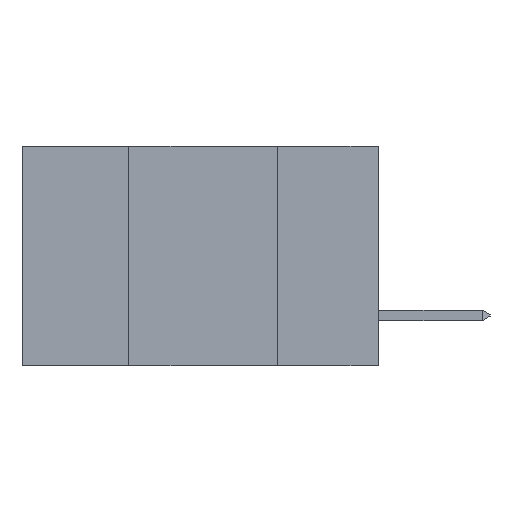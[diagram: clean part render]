
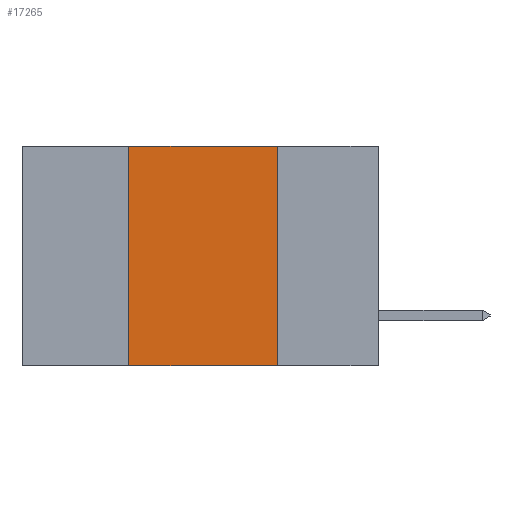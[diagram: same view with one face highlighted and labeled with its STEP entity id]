
A CAD part, left-side view. The second image highlights one B-rep face of the part: STEP entity #17265.
In plain terms, the highlighted planar face has unit normal (-1, 0, 0).
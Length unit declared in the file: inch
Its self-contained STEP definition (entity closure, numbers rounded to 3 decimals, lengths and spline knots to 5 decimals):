
#1045 = ORIENTED_EDGE ( 'NONE', *, *, #14890, .F. ) ;
#1992 = ORIENTED_EDGE ( 'NONE', *, *, #7473, .F. ) ;
#3043 = VECTOR ( 'NONE', #18909, 39.37008 ) ;
#3539 = DIRECTION ( 'NONE',  ( 0., 0., -1. ) ) ;
#3672 = PLANE ( 'NONE',  #11408 ) ;
#6373 = LINE ( 'NONE', #8031, #9972 ) ;
#6906 = CARTESIAN_POINT ( 'NONE',  ( 0., 0.6, 0. ) ) ;
#7210 = ORIENTED_EDGE ( 'NONE', *, *, #8433, .F. ) ;
#7400 = LINE ( 'NONE', #14899, #11900 ) ;
#7473 = EDGE_CURVE ( 'NONE', #14753, #12219, #7400, .T. ) ;
#8031 = CARTESIAN_POINT ( 'NONE',  ( 0., 0.17, -0.37 ) ) ;
#8240 = CARTESIAN_POINT ( 'NONE',  ( 0., 0.6, 0. ) ) ;
#8433 = EDGE_CURVE ( 'NONE', #16001, #8693, #6373, .T. ) ;
#8515 = FACE_OUTER_BOUND ( 'NONE', #13939, .T. ) ;
#8517 = CARTESIAN_POINT ( 'NONE',  ( 0., 0.6, -0.37 ) ) ;
#8693 = VERTEX_POINT ( 'NONE', #8708 ) ;
#8708 = CARTESIAN_POINT ( 'NONE',  ( 0., 0.17, -0.37 ) ) ;
#9569 = VECTOR ( 'NONE', #15900, 39.37008 ) ;
#9775 = DIRECTION ( 'NONE',  ( 0., 0., -1. ) ) ;
#9972 = VECTOR ( 'NONE', #3539, 39.37008 ) ;
#10626 = LINE ( 'NONE', #8517, #3043 ) ;
#11408 = AXIS2_PLACEMENT_3D ( 'NONE', #8240, #18656, #9775 ) ;
#11900 = VECTOR ( 'NONE', #17886, 39.37008 ) ;
#12219 = VERTEX_POINT ( 'NONE', #15940 ) ;
#13939 = EDGE_LOOP ( 'NONE', ( #7210, #1045, #1992, #17986 ) ) ;
#14753 = VERTEX_POINT ( 'NONE', #18864 ) ;
#14890 = EDGE_CURVE ( 'NONE', #12219, #16001, #17966, .T. ) ;
#14899 = CARTESIAN_POINT ( 'NONE',  ( 0., 0.42, -0.37 ) ) ;
#15900 = DIRECTION ( 'NONE',  ( 0., -1., 0. ) ) ;
#15940 = CARTESIAN_POINT ( 'NONE',  ( 0., 0.42, 0. ) ) ;
#16001 = VERTEX_POINT ( 'NONE', #18361 ) ;
#17265 = ADVANCED_FACE ( 'NONE', ( #8515 ), #3672, .F. ) ;
#17391 = EDGE_CURVE ( 'NONE', #14753, #8693, #10626, .T. ) ;
#17886 = DIRECTION ( 'NONE',  ( 0., 0., 1. ) ) ;
#17966 = LINE ( 'NONE', #6906, #9569 ) ;
#17986 = ORIENTED_EDGE ( 'NONE', *, *, #17391, .T. ) ;
#18361 = CARTESIAN_POINT ( 'NONE',  ( 0., 0.17, 0. ) ) ;
#18656 = DIRECTION ( 'NONE',  ( 1., 0., 0. ) ) ;
#18864 = CARTESIAN_POINT ( 'NONE',  ( 0., 0.42, -0.37 ) ) ;
#18909 = DIRECTION ( 'NONE',  ( 0., -1., 0. ) ) ;
